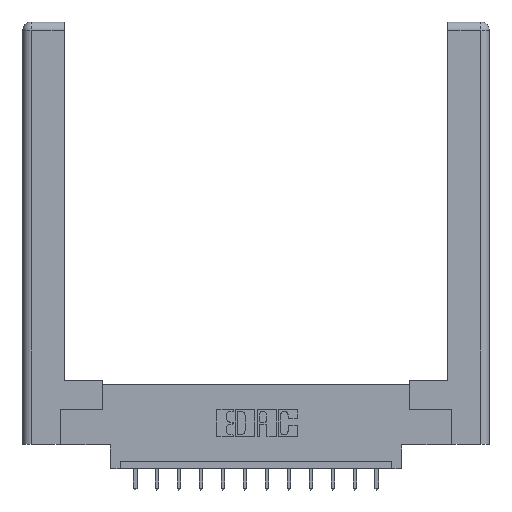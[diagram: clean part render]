
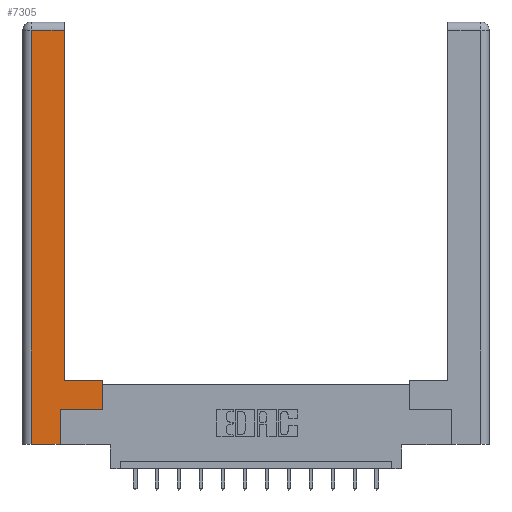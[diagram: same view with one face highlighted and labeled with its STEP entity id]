
A CAD part, top view. The second image highlights one B-rep face of the part: STEP entity #7305.
In plain terms, the highlighted planar face has unit normal (0, 0, 1).
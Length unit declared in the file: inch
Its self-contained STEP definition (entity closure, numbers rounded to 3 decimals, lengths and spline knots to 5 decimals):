
#2 = VERTEX_POINT ( 'NONE', #10600 ) ;
#182 = ORIENTED_EDGE ( 'NONE', *, *, #11691, .T. ) ;
#272 = EDGE_CURVE ( 'NONE', #4351, #14586, #9020, .T. ) ;
#638 = EDGE_LOOP ( 'NONE', ( #9714, #182, #10454, #4089, #2537, #4669, #4619, #11915 ) ) ;
#759 = CARTESIAN_POINT ( 'NONE',  ( 0.295, 0.45, 0. ) ) ;
#1000 = EDGE_CURVE ( 'NONE', #8810, #6525, #2758, .T. ) ;
#1912 = DIRECTION ( 'NONE',  ( 0., 1., 0. ) ) ;
#2214 = VECTOR ( 'NONE', #1912, 39.37008 ) ;
#2456 = DIRECTION ( 'NONE',  ( -1., 0., 0. ) ) ;
#2491 = VECTOR ( 'NONE', #2659, 39.37008 ) ;
#2537 = ORIENTED_EDGE ( 'NONE', *, *, #6547, .T. ) ;
#2574 = LINE ( 'NONE', #14856, #12539 ) ;
#2659 = DIRECTION ( 'NONE',  ( 0., 1., 0. ) ) ;
#2758 = LINE ( 'NONE', #6751, #11049 ) ;
#3003 = LINE ( 'NONE', #9849, #5636 ) ;
#3267 = LINE ( 'NONE', #759, #6076 ) ;
#3445 = LINE ( 'NONE', #7091, #2491 ) ;
#3593 = DIRECTION ( 'NONE',  ( 0., -1., 0. ) ) ;
#4089 = ORIENTED_EDGE ( 'NONE', *, *, #14921, .T. ) ;
#4351 = VERTEX_POINT ( 'NONE', #13203 ) ;
#4381 = CARTESIAN_POINT ( 'NONE',  ( 0.265, 0., 0. ) ) ;
#4616 = VERTEX_POINT ( 'NONE', #12599 ) ;
#4619 = ORIENTED_EDGE ( 'NONE', *, *, #15597, .T. ) ;
#4669 = ORIENTED_EDGE ( 'NONE', *, *, #6988, .T. ) ;
#5072 = CARTESIAN_POINT ( 'NONE',  ( 0.0615, 0., 0. ) ) ;
#5173 = CARTESIAN_POINT ( 'NONE',  ( 0.265, 0.245, 0. ) ) ;
#5561 = LINE ( 'NONE', #9078, #12335 ) ;
#5636 = VECTOR ( 'NONE', #2456, 39.37008 ) ;
#5651 = PLANE ( 'NONE',  #7519 ) ;
#6076 = VECTOR ( 'NONE', #10163, 39.37008 ) ;
#6111 = FACE_OUTER_BOUND ( 'NONE', #638, .T. ) ;
#6525 = VERTEX_POINT ( 'NONE', #5072 ) ;
#6547 = EDGE_CURVE ( 'NONE', #8640, #13098, #2574, .T. ) ;
#6751 = CARTESIAN_POINT ( 'NONE',  ( 0.0615, 0., 0. ) ) ;
#6789 = DIRECTION ( 'NONE',  ( 1., 0., 0. ) ) ;
#6791 = DIRECTION ( 'NONE',  ( 1., 0., 0. ) ) ;
#6988 = EDGE_CURVE ( 'NONE', #13098, #4616, #5561, .T. ) ;
#7045 = VECTOR ( 'NONE', #6791, 39.37008 ) ;
#7091 = CARTESIAN_POINT ( 'NONE',  ( 0.565, 0.45, 0. ) ) ;
#7305 = ADVANCED_FACE ( 'NONE', ( #6111 ), #5651, .F. ) ;
#7519 = AXIS2_PLACEMENT_3D ( 'NONE', #12720, #15144, #14071 ) ;
#7658 = DIRECTION ( 'NONE',  ( 0., 1., 0. ) ) ;
#8640 = VERTEX_POINT ( 'NONE', #13810 ) ;
#8810 = VERTEX_POINT ( 'NONE', #11680 ) ;
#9020 = LINE ( 'NONE', #10212, #2214 ) ;
#9078 = CARTESIAN_POINT ( 'NONE',  ( 0.565, 0.245, 0. ) ) ;
#9081 = EDGE_CURVE ( 'NONE', #2, #4351, #3267, .T. ) ;
#9638 = CARTESIAN_POINT ( 'NONE',  ( 0.295, 2.94, 0. ) ) ;
#9714 = ORIENTED_EDGE ( 'NONE', *, *, #272, .T. ) ;
#9849 = CARTESIAN_POINT ( 'NONE',  ( 0.0615, 2.94, 0. ) ) ;
#10163 = DIRECTION ( 'NONE',  ( -1., 0., 0. ) ) ;
#10212 = CARTESIAN_POINT ( 'NONE',  ( 0.295, 3., 0. ) ) ;
#10454 = ORIENTED_EDGE ( 'NONE', *, *, #1000, .T. ) ;
#10600 = CARTESIAN_POINT ( 'NONE',  ( 0.565, 0.45, 0. ) ) ;
#11049 = VECTOR ( 'NONE', #3593, 39.37008 ) ;
#11680 = CARTESIAN_POINT ( 'NONE',  ( 0.0615, 2.94, 0. ) ) ;
#11691 = EDGE_CURVE ( 'NONE', #14586, #8810, #3003, .T. ) ;
#11915 = ORIENTED_EDGE ( 'NONE', *, *, #9081, .T. ) ;
#12335 = VECTOR ( 'NONE', #6789, 39.37008 ) ;
#12539 = VECTOR ( 'NONE', #7658, 39.37008 ) ;
#12599 = CARTESIAN_POINT ( 'NONE',  ( 0.565, 0.245, 0. ) ) ;
#12720 = CARTESIAN_POINT ( 'NONE',  ( 0., 0., 0. ) ) ;
#13098 = VERTEX_POINT ( 'NONE', #5173 ) ;
#13203 = CARTESIAN_POINT ( 'NONE',  ( 0.295, 0.45, 0. ) ) ;
#13810 = CARTESIAN_POINT ( 'NONE',  ( 0.265, 0., 0. ) ) ;
#13817 = LINE ( 'NONE', #4381, #7045 ) ;
#14071 = DIRECTION ( 'NONE',  ( -1., 0., 0. ) ) ;
#14586 = VERTEX_POINT ( 'NONE', #9638 ) ;
#14856 = CARTESIAN_POINT ( 'NONE',  ( 0.265, 0.245, 0. ) ) ;
#14921 = EDGE_CURVE ( 'NONE', #6525, #8640, #13817, .T. ) ;
#15144 = DIRECTION ( 'NONE',  ( 0., 0., -1. ) ) ;
#15597 = EDGE_CURVE ( 'NONE', #4616, #2, #3445, .T. ) ;
